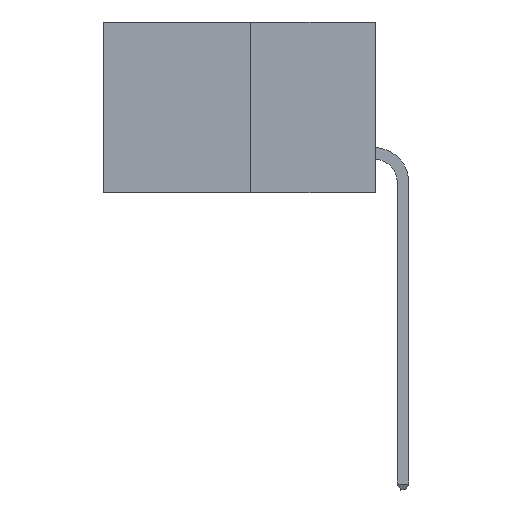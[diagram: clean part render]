
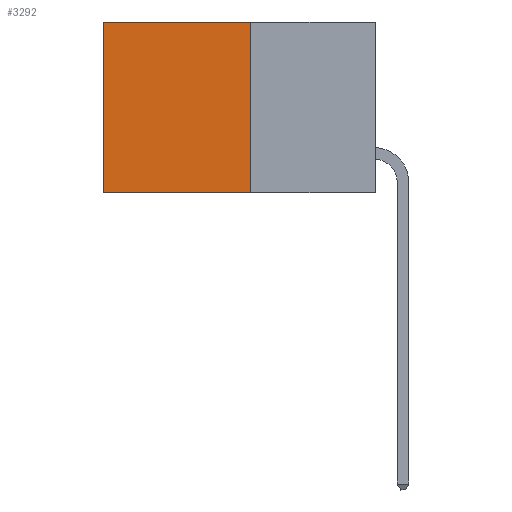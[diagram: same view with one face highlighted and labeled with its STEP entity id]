
A CAD part, left-side view. The second image highlights one B-rep face of the part: STEP entity #3292.
In plain terms, the highlighted planar face has unit normal (-1, 0, 0).
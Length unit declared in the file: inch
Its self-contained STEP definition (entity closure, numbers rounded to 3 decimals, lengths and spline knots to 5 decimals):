
#131 = LINE ( 'NONE', #10403, #12702 ) ;
#393 = DIRECTION ( 'NONE',  ( 0., 1., 0. ) ) ;
#643 = ORIENTED_EDGE ( 'NONE', *, *, #10565, .T. ) ;
#1102 = DIRECTION ( 'NONE',  ( 0., 0., -1. ) ) ;
#1137 = VECTOR ( 'NONE', #9285, 39.37008 ) ;
#1224 = CARTESIAN_POINT ( 'NONE',  ( 0.277, 0.27, -0.37 ) ) ;
#1845 = VECTOR ( 'NONE', #10161, 39.37008 ) ;
#2108 = VERTEX_POINT ( 'NONE', #5074 ) ;
#2515 = CARTESIAN_POINT ( 'NONE',  ( 0.277, 0.27, -0.37 ) ) ;
#3063 = EDGE_CURVE ( 'NONE', #2108, #3800, #9794, .T. ) ;
#3292 = ADVANCED_FACE ( 'NONE', ( #4757 ), #6437, .F. ) ;
#3367 = CARTESIAN_POINT ( 'NONE',  ( 0.277, 0.59, -0.37 ) ) ;
#3740 = LINE ( 'NONE', #1224, #5452 ) ;
#3794 = ORIENTED_EDGE ( 'NONE', *, *, #5670, .F. ) ;
#3800 = VERTEX_POINT ( 'NONE', #7461 ) ;
#3943 = LINE ( 'NONE', #3367, #1137 ) ;
#4757 = FACE_OUTER_BOUND ( 'NONE', #5837, .T. ) ;
#5074 = CARTESIAN_POINT ( 'NONE',  ( 0.277, 0.27, -0.37 ) ) ;
#5161 = CARTESIAN_POINT ( 'NONE',  ( 0.277, 0.27, 0. ) ) ;
#5452 = VECTOR ( 'NONE', #1102, 39.37008 ) ;
#5670 = EDGE_CURVE ( 'NONE', #11683, #2108, #3740, .T. ) ;
#5835 = DIRECTION ( 'NONE',  ( 0., 0., -1. ) ) ;
#5837 = EDGE_LOOP ( 'NONE', ( #643, #11265, #3794, #7054 ) ) ;
#6422 = DIRECTION ( 'NONE',  ( 1., 0., 0. ) ) ;
#6437 = PLANE ( 'NONE',  #8768 ) ;
#6691 = CARTESIAN_POINT ( 'NONE',  ( 0.277, 0.27, -0.37 ) ) ;
#6833 = VERTEX_POINT ( 'NONE', #9687 ) ;
#7054 = ORIENTED_EDGE ( 'NONE', *, *, #10669, .T. ) ;
#7461 = CARTESIAN_POINT ( 'NONE',  ( 0.277, 0.59, -0.37 ) ) ;
#8768 = AXIS2_PLACEMENT_3D ( 'NONE', #6691, #6422, #5835 ) ;
#9285 = DIRECTION ( 'NONE',  ( 0., 0., -1. ) ) ;
#9687 = CARTESIAN_POINT ( 'NONE',  ( 0.277, 0.59, 0. ) ) ;
#9794 = LINE ( 'NONE', #2515, #1845 ) ;
#10161 = DIRECTION ( 'NONE',  ( 0., 1., 0. ) ) ;
#10403 = CARTESIAN_POINT ( 'NONE',  ( 0.277, 0.27, 0. ) ) ;
#10565 = EDGE_CURVE ( 'NONE', #6833, #3800, #3943, .T. ) ;
#10669 = EDGE_CURVE ( 'NONE', #11683, #6833, #131, .T. ) ;
#11265 = ORIENTED_EDGE ( 'NONE', *, *, #3063, .F. ) ;
#11683 = VERTEX_POINT ( 'NONE', #5161 ) ;
#12702 = VECTOR ( 'NONE', #393, 39.37008 ) ;
